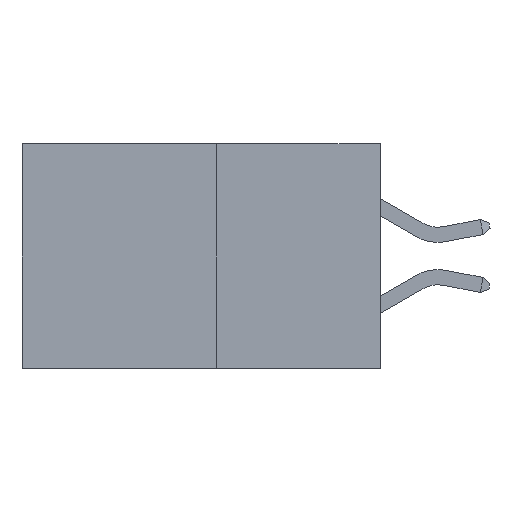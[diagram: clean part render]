
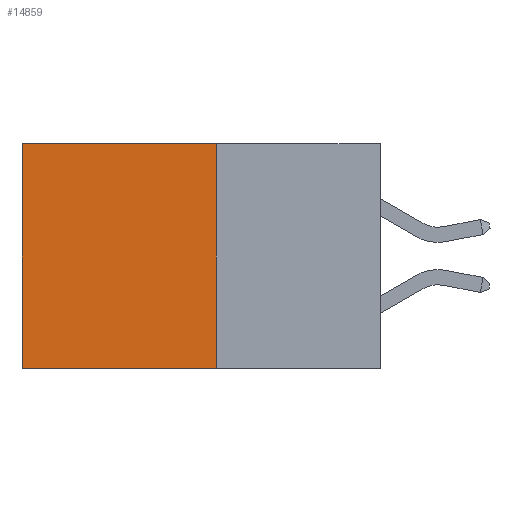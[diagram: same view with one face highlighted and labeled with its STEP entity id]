
A CAD part, left-side view. The second image highlights one B-rep face of the part: STEP entity #14859.
In plain terms, the highlighted planar face has unit normal (-1, 0, 0).
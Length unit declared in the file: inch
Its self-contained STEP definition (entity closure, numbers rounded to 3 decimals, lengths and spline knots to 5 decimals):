
#454 = LINE ( 'NONE', #2410, #7324 ) ;
#614 = VERTEX_POINT ( 'NONE', #12981 ) ;
#1249 = PLANE ( 'NONE',  #16147 ) ;
#1544 = ORIENTED_EDGE ( 'NONE', *, *, #14879, .F. ) ;
#2341 = ORIENTED_EDGE ( 'NONE', *, *, #14822, .T. ) ;
#2410 = CARTESIAN_POINT ( 'NONE',  ( 0.277, 0.27, 0. ) ) ;
#2527 = DIRECTION ( 'NONE',  ( 1., 0., 0. ) ) ;
#3060 = VECTOR ( 'NONE', #6488, 39.37008 ) ;
#3288 = CARTESIAN_POINT ( 'NONE',  ( 0.277, 0.27, -0.37 ) ) ;
#3516 = EDGE_LOOP ( 'NONE', ( #9840, #10236, #1544, #2341 ) ) ;
#3952 = EDGE_CURVE ( 'NONE', #6351, #6389, #6135, .T. ) ;
#6092 = LINE ( 'NONE', #14166, #3060 ) ;
#6135 = LINE ( 'NONE', #3288, #9589 ) ;
#6351 = VERTEX_POINT ( 'NONE', #15024 ) ;
#6389 = VERTEX_POINT ( 'NONE', #12497 ) ;
#6488 = DIRECTION ( 'NONE',  ( 0., 0., -1. ) ) ;
#7098 = LINE ( 'NONE', #16006, #13525 ) ;
#7324 = VECTOR ( 'NONE', #11528, 39.37008 ) ;
#8844 = CARTESIAN_POINT ( 'NONE',  ( 0.277, 0.27, 0. ) ) ;
#8993 = CARTESIAN_POINT ( 'NONE',  ( 0.277, 0.27, -0.37 ) ) ;
#9589 = VECTOR ( 'NONE', #15307, 39.37008 ) ;
#9803 = EDGE_CURVE ( 'NONE', #614, #6389, #7098, .T. ) ;
#9840 = ORIENTED_EDGE ( 'NONE', *, *, #9803, .T. ) ;
#10236 = ORIENTED_EDGE ( 'NONE', *, *, #3952, .F. ) ;
#11528 = DIRECTION ( 'NONE',  ( 0., 1., 0. ) ) ;
#11595 = DIRECTION ( 'NONE',  ( 0., 0., -1. ) ) ;
#11885 = VERTEX_POINT ( 'NONE', #8844 ) ;
#12497 = CARTESIAN_POINT ( 'NONE',  ( 0.277, 0.59, -0.37 ) ) ;
#12981 = CARTESIAN_POINT ( 'NONE',  ( 0.277, 0.59, 0. ) ) ;
#13525 = VECTOR ( 'NONE', #16166, 39.37008 ) ;
#14166 = CARTESIAN_POINT ( 'NONE',  ( 0.277, 0.27, -0.37 ) ) ;
#14822 = EDGE_CURVE ( 'NONE', #11885, #614, #454, .T. ) ;
#14859 = ADVANCED_FACE ( 'NONE', ( #16184 ), #1249, .F. ) ;
#14879 = EDGE_CURVE ( 'NONE', #11885, #6351, #6092, .T. ) ;
#15024 = CARTESIAN_POINT ( 'NONE',  ( 0.277, 0.27, -0.37 ) ) ;
#15307 = DIRECTION ( 'NONE',  ( 0., 1., 0. ) ) ;
#16006 = CARTESIAN_POINT ( 'NONE',  ( 0.277, 0.59, -0.37 ) ) ;
#16147 = AXIS2_PLACEMENT_3D ( 'NONE', #8993, #2527, #11595 ) ;
#16166 = DIRECTION ( 'NONE',  ( 0., 0., -1. ) ) ;
#16184 = FACE_OUTER_BOUND ( 'NONE', #3516, .T. ) ;
